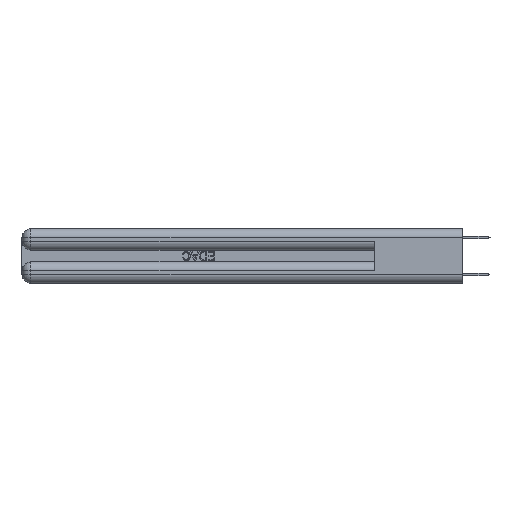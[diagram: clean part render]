
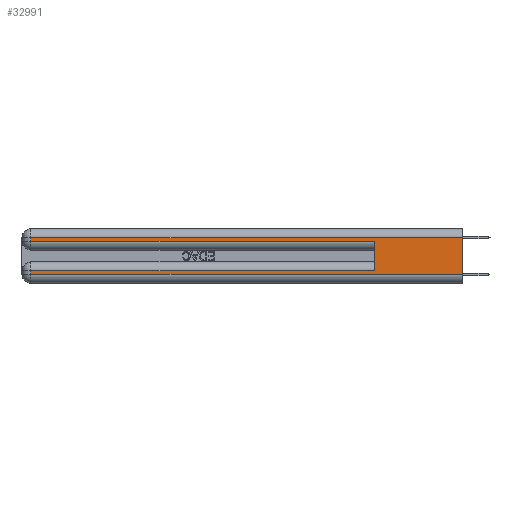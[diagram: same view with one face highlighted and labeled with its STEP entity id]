
A CAD part, left-side view. The second image highlights one B-rep face of the part: STEP entity #32991.
In plain terms, the highlighted planar face has unit normal (-1, 0, 0).
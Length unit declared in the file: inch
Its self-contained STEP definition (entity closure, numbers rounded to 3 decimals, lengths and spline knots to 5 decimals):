
#181 = LINE ( 'NONE', #8122, #16997 ) ;
#259 = DIRECTION ( 'NONE',  ( 0., 0., 1. ) ) ;
#371 = ORIENTED_EDGE ( 'NONE', *, *, #27983, .F. ) ;
#582 = LINE ( 'NONE', #17527, #24585 ) ;
#613 = LINE ( 'NONE', #11614, #28985 ) ;
#779 = CARTESIAN_POINT ( 'NONE',  ( 0., 0., 0.085 ) ) ;
#840 = CARTESIAN_POINT ( 'NONE',  ( 0., 2.94, 0.085 ) ) ;
#1590 = LINE ( 'NONE', #32323, #20074 ) ;
#2075 = ORIENTED_EDGE ( 'NONE', *, *, #24576, .T. ) ;
#2144 = DIRECTION ( 'NONE',  ( 0., 1., 0. ) ) ;
#3783 = VERTEX_POINT ( 'NONE', #31889 ) ;
#5060 = VERTEX_POINT ( 'NONE', #840 ) ;
#5983 = CARTESIAN_POINT ( 'NONE',  ( 0., 0., 0.37 ) ) ;
#6178 = LINE ( 'NONE', #779, #8167 ) ;
#6583 = CARTESIAN_POINT ( 'NONE',  ( 0., 2.94, 0.31 ) ) ;
#8122 = CARTESIAN_POINT ( 'NONE',  ( 0., 0., 0.06 ) ) ;
#8167 = VECTOR ( 'NONE', #11778, 39.37008 ) ;
#8909 = VECTOR ( 'NONE', #28150, 39.37008 ) ;
#9834 = VERTEX_POINT ( 'NONE', #31581 ) ;
#10048 = DIRECTION ( 'NONE',  ( 0., 0., -1. ) ) ;
#10687 = EDGE_CURVE ( 'NONE', #5060, #9834, #582, .T. ) ;
#11614 = CARTESIAN_POINT ( 'NONE',  ( 0., 0.6, 0.145 ) ) ;
#11778 = DIRECTION ( 'NONE',  ( 0., 1., 0. ) ) ;
#12287 = ORIENTED_EDGE ( 'NONE', *, *, #21939, .T. ) ;
#12679 = VECTOR ( 'NONE', #2144, 39.37008 ) ;
#12756 = CARTESIAN_POINT ( 'NONE',  ( 0., 0.6, 0.285 ) ) ;
#13676 = ORIENTED_EDGE ( 'NONE', *, *, #17024, .F. ) ;
#13794 = CARTESIAN_POINT ( 'NONE',  ( 0., 2.94, 0.37 ) ) ;
#13901 = CARTESIAN_POINT ( 'NONE',  ( 0., 0., 0.31 ) ) ;
#13965 = DIRECTION ( 'NONE',  ( 0., 0., -1. ) ) ;
#14204 = EDGE_LOOP ( 'NONE', ( #13676, #26332, #16000, #2075, #371, #12287, #31324, #30712 ) ) ;
#15315 = CARTESIAN_POINT ( 'NONE',  ( 0., 0., 0.31 ) ) ;
#15382 = VERTEX_POINT ( 'NONE', #13901 ) ;
#16000 = ORIENTED_EDGE ( 'NONE', *, *, #23176, .T. ) ;
#16288 = VECTOR ( 'NONE', #13965, 39.37008 ) ;
#16302 = AXIS2_PLACEMENT_3D ( 'NONE', #5983, #28075, #19539 ) ;
#16997 = VECTOR ( 'NONE', #22199, 39.37008 ) ;
#17024 = EDGE_CURVE ( 'NONE', #15382, #19848, #1590, .T. ) ;
#17089 = LINE ( 'NONE', #22321, #8909 ) ;
#17105 = VERTEX_POINT ( 'NONE', #12756 ) ;
#17356 = DIRECTION ( 'NONE',  ( 0., 0., -1. ) ) ;
#17527 = CARTESIAN_POINT ( 'NONE',  ( 0., 2.94, 0.37 ) ) ;
#19539 = DIRECTION ( 'NONE',  ( 0., 0., -1. ) ) ;
#19676 = CARTESIAN_POINT ( 'NONE',  ( 0., 0., 0.06 ) ) ;
#19848 = VERTEX_POINT ( 'NONE', #19676 ) ;
#20074 = VECTOR ( 'NONE', #10048, 39.37008 ) ;
#21939 = EDGE_CURVE ( 'NONE', #3783, #5060, #6178, .T. ) ;
#22199 = DIRECTION ( 'NONE',  ( 0., -1., 0. ) ) ;
#22274 = LINE ( 'NONE', #13794, #16288 ) ;
#22321 = CARTESIAN_POINT ( 'NONE',  ( 0., 0., 0.285 ) ) ;
#23176 = EDGE_CURVE ( 'NONE', #26794, #28888, #22274, .T. ) ;
#24576 = EDGE_CURVE ( 'NONE', #28888, #17105, #17089, .T. ) ;
#24585 = VECTOR ( 'NONE', #17356, 39.37008 ) ;
#25504 = FACE_OUTER_BOUND ( 'NONE', #14204, .T. ) ;
#25572 = EDGE_CURVE ( 'NONE', #15382, #26794, #32176, .T. ) ;
#26332 = ORIENTED_EDGE ( 'NONE', *, *, #25572, .T. ) ;
#26750 = CARTESIAN_POINT ( 'NONE',  ( 0., 2.94, 0.285 ) ) ;
#26794 = VERTEX_POINT ( 'NONE', #6583 ) ;
#27983 = EDGE_CURVE ( 'NONE', #3783, #17105, #613, .T. ) ;
#28075 = DIRECTION ( 'NONE',  ( 1., 0., 0. ) ) ;
#28150 = DIRECTION ( 'NONE',  ( 0., -1., 0. ) ) ;
#28888 = VERTEX_POINT ( 'NONE', #26750 ) ;
#28920 = PLANE ( 'NONE',  #16302 ) ;
#28985 = VECTOR ( 'NONE', #259, 39.37008 ) ;
#30712 = ORIENTED_EDGE ( 'NONE', *, *, #31601, .T. ) ;
#31324 = ORIENTED_EDGE ( 'NONE', *, *, #10687, .T. ) ;
#31581 = CARTESIAN_POINT ( 'NONE',  ( 0., 2.94, 0.06 ) ) ;
#31601 = EDGE_CURVE ( 'NONE', #9834, #19848, #181, .T. ) ;
#31889 = CARTESIAN_POINT ( 'NONE',  ( 0., 0.6, 0.085 ) ) ;
#32176 = LINE ( 'NONE', #15315, #12679 ) ;
#32323 = CARTESIAN_POINT ( 'NONE',  ( 0., 0., 0.37 ) ) ;
#32991 = ADVANCED_FACE ( 'NONE', ( #25504 ), #28920, .F. ) ;
